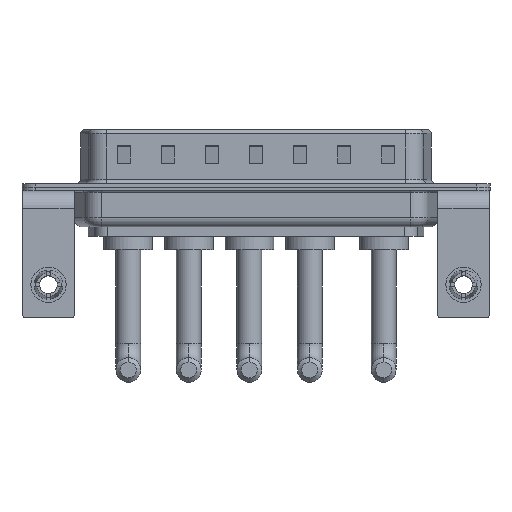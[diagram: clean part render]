
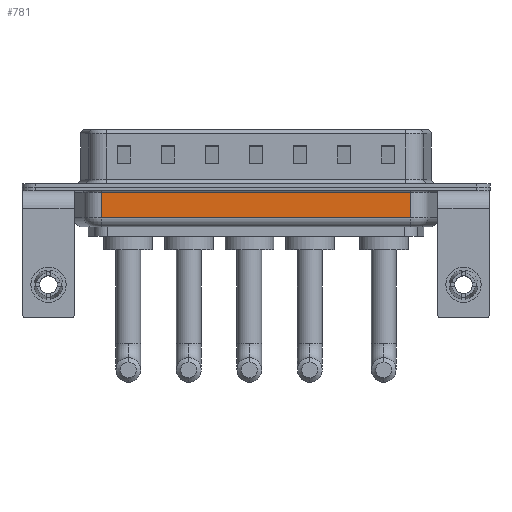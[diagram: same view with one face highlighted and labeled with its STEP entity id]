
A CAD part, front view. The second image highlights one B-rep face of the part: STEP entity #781.
In plain terms, the highlighted planar face has unit normal (0, -1, 0).
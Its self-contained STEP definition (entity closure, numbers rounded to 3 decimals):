
#526 = ORIENTED_EDGE ( 'NONE', *, *, #6940, .F. ) ;
#781 = ADVANCED_FACE ( 'NONE', ( #2211 ), #16079, .F. ) ;
#1859 = CARTESIAN_POINT ( 'NONE',  ( 6.006, -5.35, -0.65 ) ) ;
#2211 = FACE_OUTER_BOUND ( 'NONE', #7917, .T. ) ;
#3039 = CARTESIAN_POINT ( 'NONE',  ( 6.006, -5.35, -0.65 ) ) ;
#3412 = VECTOR ( 'NONE', #14047, 1000. ) ;
#3413 = LINE ( 'NONE', #16488, #12929 ) ;
#3665 = DIRECTION ( 'NONE',  ( 0., 0., 1. ) ) ;
#3837 = VERTEX_POINT ( 'NONE', #15297 ) ;
#4278 = EDGE_CURVE ( 'NONE', #12205, #16270, #13721, .T. ) ;
#4291 = DIRECTION ( 'NONE',  ( 0., 1., 0. ) ) ;
#4328 = AXIS2_PLACEMENT_3D ( 'NONE', #9847, #4291, #9529 ) ;
#4468 = ORIENTED_EDGE ( 'NONE', *, *, #11276, .T. ) ;
#5673 = ORIENTED_EDGE ( 'NONE', *, *, #4278, .T. ) ;
#6047 = VECTOR ( 'NONE', #15109, 1000. ) ;
#6940 = EDGE_CURVE ( 'NONE', #12205, #13201, #10090, .T. ) ;
#7917 = EDGE_LOOP ( 'NONE', ( #526, #5673, #11478, #4468 ) ) ;
#8201 = LINE ( 'NONE', #1859, #16674 ) ;
#9529 = DIRECTION ( 'NONE',  ( 0., 0., 1. ) ) ;
#9847 = CARTESIAN_POINT ( 'NONE',  ( 6.006, -5.35, -4.5 ) ) ;
#10090 = LINE ( 'NONE', #11469, #3412 ) ;
#11276 = EDGE_CURVE ( 'NONE', #3837, #13201, #8201, .T. ) ;
#11469 = CARTESIAN_POINT ( 'NONE',  ( 6.006, -5.35, -4.5 ) ) ;
#11478 = ORIENTED_EDGE ( 'NONE', *, *, #16606, .T. ) ;
#12205 = VERTEX_POINT ( 'NONE', #14706 ) ;
#12929 = VECTOR ( 'NONE', #3665, 1000. ) ;
#13201 = VERTEX_POINT ( 'NONE', #3039 ) ;
#13721 = LINE ( 'NONE', #14055, #6047 ) ;
#14047 = DIRECTION ( 'NONE',  ( 0., 0., 1. ) ) ;
#14055 = CARTESIAN_POINT ( 'NONE',  ( 6.006, -5.35, -3.5 ) ) ;
#14344 = CARTESIAN_POINT ( 'NONE',  ( 41.044, -5.35, -3.5 ) ) ;
#14706 = CARTESIAN_POINT ( 'NONE',  ( 6.006, -5.35, -3.5 ) ) ;
#15109 = DIRECTION ( 'NONE',  ( 1., 0., 0. ) ) ;
#15297 = CARTESIAN_POINT ( 'NONE',  ( 41.044, -5.35, -0.65 ) ) ;
#15968 = DIRECTION ( 'NONE',  ( -1., 0., 0. ) ) ;
#16079 = PLANE ( 'NONE',  #4328 ) ;
#16270 = VERTEX_POINT ( 'NONE', #14344 ) ;
#16488 = CARTESIAN_POINT ( 'NONE',  ( 41.044, -5.35, -4.5 ) ) ;
#16606 = EDGE_CURVE ( 'NONE', #16270, #3837, #3413, .T. ) ;
#16674 = VECTOR ( 'NONE', #15968, 1000. ) ;
